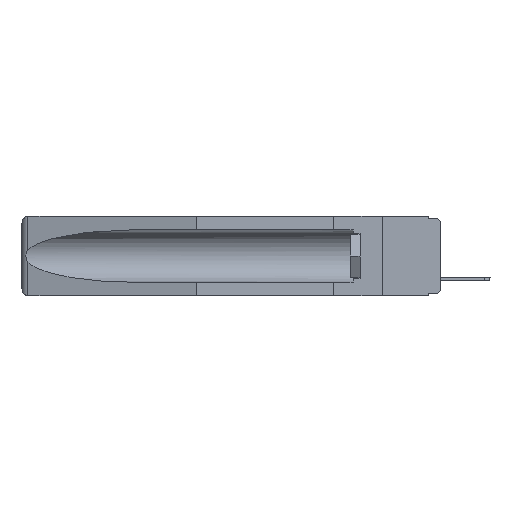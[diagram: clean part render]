
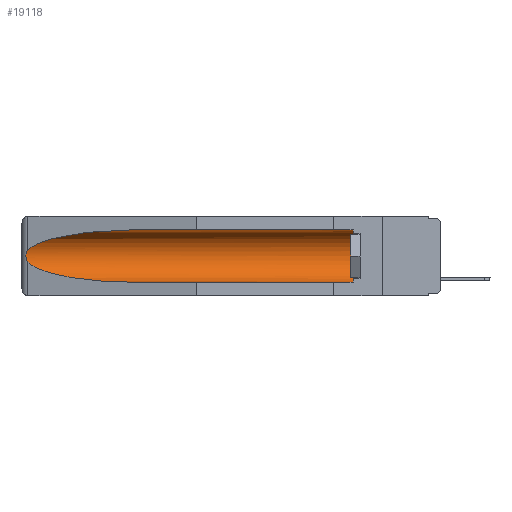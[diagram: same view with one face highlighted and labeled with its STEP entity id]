
A CAD part, left-side view. The second image highlights one B-rep face of the part: STEP entity #19118.
In plain terms, the highlighted cylindrical face has radius 2.857 mm (diameter 5.715 mm), a partial arc.
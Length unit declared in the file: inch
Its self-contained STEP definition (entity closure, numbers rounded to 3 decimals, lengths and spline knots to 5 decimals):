
#189 = DIRECTION ( 'NONE',  ( 0., 0., 1. ) ) ;
#915 = ORIENTED_EDGE ( 'NONE', *, *, #1177, .T. ) ;
#1177 = EDGE_CURVE ( 'NONE', #1656, #16398, #18787, .T. ) ;
#1607 = ORIENTED_EDGE ( 'NONE', *, *, #8827, .T. ) ;
#1656 = VERTEX_POINT ( 'NONE', #16642 ) ;
#2161 = CARTESIAN_POINT ( 'NONE',  ( 0.2675, 1.53308, -0.16763 ) ) ;
#2294 = CARTESIAN_POINT ( 'NONE',  ( 0.26597, 1.52961, -0.15275 ) ) ;
#2300 = CARTESIAN_POINT ( 'NONE',  ( 0.155, 0.126, -0.1715 ) ) ;
#2381 = CARTESIAN_POINT ( 'NONE',  ( 0.26537, 1.52718, -0.14972 ) ) ;
#3486 = B_SPLINE_CURVE_WITH_KNOTS ( 'NONE', 3,
 ( #6603, #2294, #10650, #4384, #2161, #16168, #8435, #10261, #16432, #18295 ),
 .UNSPECIFIED., .F., .F.,
 ( 4, 2, 2, 2, 4 ),
 ( 0., 0.00029, 0.00058, 0.00087, 0.00117 ),
 .UNSPECIFIED. ) ;
#4384 = CARTESIAN_POINT ( 'NONE',  ( 0.2673, 1.5327, -0.16383 ) ) ;
#5719 = CARTESIAN_POINT ( 'NONE',  ( 0.155, 1.07973, -0.284 ) ) ;
#6510 = CYLINDRICAL_SURFACE ( 'NONE', #7068, 0.1125 ) ;
#6573 = VERTEX_POINT ( 'NONE', #18889 ) ;
#6586 = CARTESIAN_POINT ( 'NONE',  ( 0.26537, 1.52718, -0.19328 ) ) ;
#6603 = CARTESIAN_POINT ( 'NONE',  ( 0.26537, 1.52718, -0.14972 ) ) ;
#6829 = CARTESIAN_POINT ( 'NONE',  ( 0.155, -0.30754, -0.059 ) ) ;
#7068 = AXIS2_PLACEMENT_3D ( 'NONE', #8212, #14612, #14494 ) ;
#7772 = LINE ( 'NONE', #21949, #18526 ) ;
#8212 = CARTESIAN_POINT ( 'NONE',  ( 0.155, -0.30754, -0.1715 ) ) ;
#8254 = VERTEX_POINT ( 'NONE', #17389 ) ;
#8435 = CARTESIAN_POINT ( 'NONE',  ( 0.2673, 1.53269, -0.17917 ) ) ;
#8635 = EDGE_CURVE ( 'NONE', #16637, #9777, #7772, .T. ) ;
#8827 = EDGE_CURVE ( 'NONE', #16398, #8254, #10972, .T. ) ;
#9777 = VERTEX_POINT ( 'NONE', #14489 ) ;
#10261 = CARTESIAN_POINT ( 'NONE',  ( 0.26655, 1.53094, -0.18657 ) ) ;
#10493 = ORIENTED_EDGE ( 'NONE', *, *, #8635, .F. ) ;
#10644 = ORIENTED_EDGE ( 'NONE', *, *, #19528, .T. ) ;
#10650 = CARTESIAN_POINT ( 'NONE',  ( 0.26654, 1.53092, -0.15636 ) ) ;
#10678 = CIRCLE ( 'NONE', #17397, 0.1125 ) ;
#10972 =( BOUNDED_CURVE ( )  B_SPLINE_CURVE ( 3, ( #20219, #13914, #16253, #2381 ),
 .UNSPECIFIED., .F., .F. ) 
 B_SPLINE_CURVE_WITH_KNOTS ( ( 4, 4 ),
 ( 4.71239, 6.08839 ),
 .UNSPECIFIED. ) 
 CURVE ( )  GEOMETRIC_REPRESENTATION_ITEM ( )  RATIONAL_B_SPLINE_CURVE ( ( 1., 0.848, 0.848, 1. ) ) 
 REPRESENTATION_ITEM ( '' )  );
#12086 = DIRECTION ( 'NONE',  ( 0., 1., 0. ) ) ;
#12111 = DIRECTION ( 'NONE',  ( 0., -1., 0. ) ) ;
#13826 = EDGE_CURVE ( 'NONE', #16637, #1656, #10678, .T. ) ;
#13914 = CARTESIAN_POINT ( 'NONE',  ( 0.21114, 1.30732, -0.059 ) ) ;
#14489 = CARTESIAN_POINT ( 'NONE',  ( 0.155, 1.07973, -0.284 ) ) ;
#14494 = DIRECTION ( 'NONE',  ( 0., 0., 1. ) ) ;
#14612 = DIRECTION ( 'NONE',  ( 0., 1., 0. ) ) ;
#14815 = DIRECTION ( 'NONE',  ( 0., 1., 0. ) ) ;
#15772 = CARTESIAN_POINT ( 'NONE',  ( 0.155, 0.126, -0.284 ) ) ;
#16168 = CARTESIAN_POINT ( 'NONE',  ( 0.2675, 1.53308, -0.17534 ) ) ;
#16253 = CARTESIAN_POINT ( 'NONE',  ( 0.25451, 1.48313, -0.09465 ) ) ;
#16398 = VERTEX_POINT ( 'NONE', #22383 ) ;
#16424 = ORIENTED_EDGE ( 'NONE', *, *, #13826, .T. ) ;
#16432 = CARTESIAN_POINT ( 'NONE',  ( 0.26597, 1.5296, -0.19026 ) ) ;
#16550 = CARTESIAN_POINT ( 'NONE',  ( 0.25451, 1.48313, -0.24835 ) ) ;
#16637 = VERTEX_POINT ( 'NONE', #15772 ) ;
#16642 = CARTESIAN_POINT ( 'NONE',  ( 0.155, 0.126, -0.059 ) ) ;
#17389 = CARTESIAN_POINT ( 'NONE',  ( 0.26537, 1.52718, -0.14972 ) ) ;
#17397 = AXIS2_PLACEMENT_3D ( 'NONE', #2300, #12111, #189 ) ;
#18295 = CARTESIAN_POINT ( 'NONE',  ( 0.26537, 1.52718, -0.19328 ) ) ;
#18526 = VECTOR ( 'NONE', #12086, 39.37008 ) ;
#18787 = LINE ( 'NONE', #6829, #25475 ) ;
#18889 = CARTESIAN_POINT ( 'NONE',  ( 0.26537, 1.52718, -0.19328 ) ) ;
#19118 = ADVANCED_FACE ( 'NONE', ( #20551 ), #6510, .F. ) ;
#19528 = EDGE_CURVE ( 'NONE', #8254, #6573, #3486, .T. ) ;
#20219 = CARTESIAN_POINT ( 'NONE',  ( 0.155, 1.07973, -0.059 ) ) ;
#20551 = FACE_OUTER_BOUND ( 'NONE', #23296, .T. ) ;
#21124 = ORIENTED_EDGE ( 'NONE', *, *, #25895, .T. ) ;
#21949 = CARTESIAN_POINT ( 'NONE',  ( 0.155, -0.30754, -0.284 ) ) ;
#22383 = CARTESIAN_POINT ( 'NONE',  ( 0.155, 1.07973, -0.059 ) ) ;
#23296 = EDGE_LOOP ( 'NONE', ( #1607, #10644, #21124, #10493, #16424, #915 ) ) ;
#24593 = CARTESIAN_POINT ( 'NONE',  ( 0.21114, 1.30732, -0.284 ) ) ;
#25443 =( BOUNDED_CURVE ( )  B_SPLINE_CURVE ( 3, ( #6586, #16550, #24593, #5719 ),
 .UNSPECIFIED., .F., .F. ) 
 B_SPLINE_CURVE_WITH_KNOTS ( ( 4, 4 ),
 ( 0.1948, 1.5708 ),
 .UNSPECIFIED. ) 
 CURVE ( )  GEOMETRIC_REPRESENTATION_ITEM ( )  RATIONAL_B_SPLINE_CURVE ( ( 1., 0.848, 0.848, 1. ) ) 
 REPRESENTATION_ITEM ( '' )  );
#25475 = VECTOR ( 'NONE', #14815, 39.37008 ) ;
#25895 = EDGE_CURVE ( 'NONE', #6573, #9777, #25443, .T. ) ;
